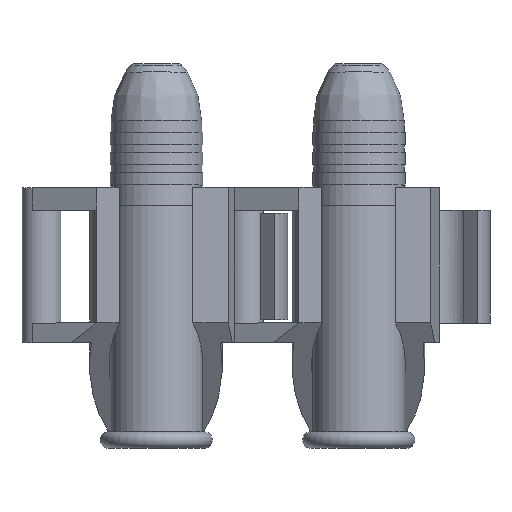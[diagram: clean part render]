
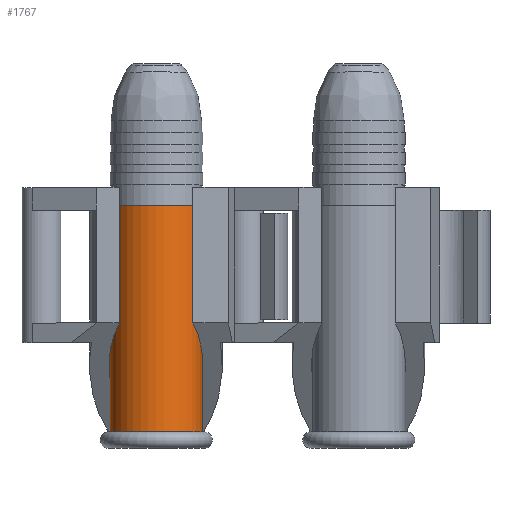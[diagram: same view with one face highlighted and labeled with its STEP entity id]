
A CAD part, top view. The second image highlights one B-rep face of the part: STEP entity #1767.
In plain terms, the highlighted cylindrical face has radius 2.845 mm (diameter 5.69 mm), a full revolution.
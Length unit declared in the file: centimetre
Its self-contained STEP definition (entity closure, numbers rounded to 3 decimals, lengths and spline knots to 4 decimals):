
#399=FACE_BOUND($,#654,.T.);
#511=FACE_OUTER_BOUND($,#653,.T.);
#653=EDGE_LOOP($,(#1599));
#654=EDGE_LOOP($,(#1600));
#761=CIRCLE($,#1970,0.2845);
#762=CIRCLE($,#1971,0.2845);
#926=VERTEX_POINT($,#3050);
#927=VERTEX_POINT($,#3052);
#1157=EDGE_CURVE($,#926,#926,#761,.T.);
#1158=EDGE_CURVE($,#927,#927,#762,.T.);
#1599=ORIENTED_EDGE($,*,*,#1157,.T.);
#1600=ORIENTED_EDGE($,*,*,#1158,.F.);
#1665=CYLINDRICAL_SURFACE($,#1969,0.2845);
#1767=ADVANCED_FACE($,(#511,#399),#1665,.T.);
#1969=AXIS2_PLACEMENT_3D($,#3049,#2483,#2484);
#1970=AXIS2_PLACEMENT_3D($,#3051,#2485,#2486);
#1971=AXIS2_PLACEMENT_3D($,#3053,#2487,#2488);
#2483=DIRECTION('center_axis',(0.,-1.,0.));
#2484=DIRECTION('ref_axis',(0.,0.,-1.));
#2485=DIRECTION('center_axis',(0.,-1.,0.));
#2486=DIRECTION('ref_axis',(0.,0.,-1.));
#2487=DIRECTION('center_axis',(0.,-1.,0.));
#2488=DIRECTION('ref_axis',(0.,0.,-1.));
#3049=CARTESIAN_POINT('Origin',(0.0016,0.02,
-0.0214));
#3050=CARTESIAN_POINT('',(0.0016,1.5186,0.263));
#3051=CARTESIAN_POINT('Origin',(0.0016,1.5186,-0.0214));
#3052=CARTESIAN_POINT('',(0.0016,0.1216,0.263));
#3053=CARTESIAN_POINT('Origin',(0.0016,0.1216,-0.0214));
